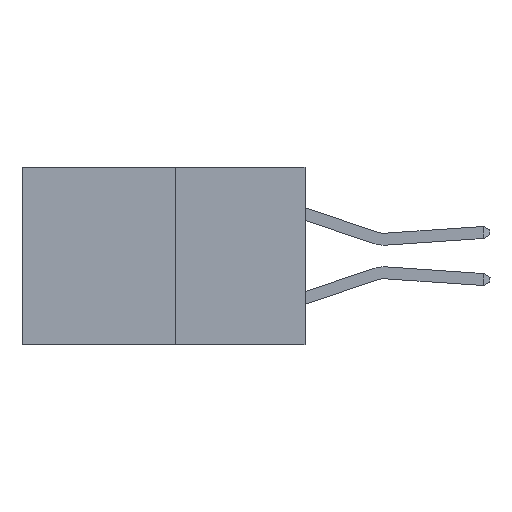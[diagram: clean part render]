
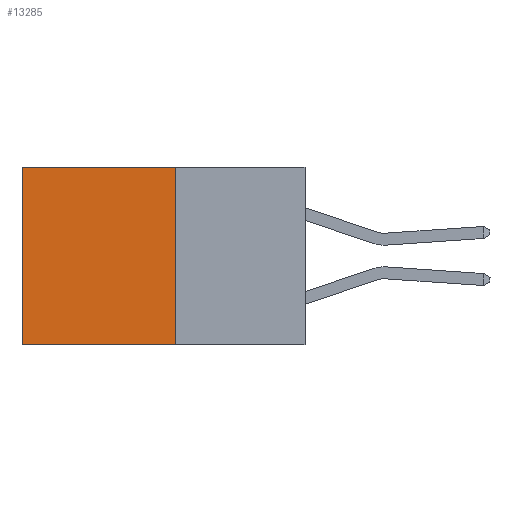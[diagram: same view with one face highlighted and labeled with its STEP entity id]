
A CAD part, left-side view. The second image highlights one B-rep face of the part: STEP entity #13285.
In plain terms, the highlighted planar face has unit normal (-1, 0, 0).
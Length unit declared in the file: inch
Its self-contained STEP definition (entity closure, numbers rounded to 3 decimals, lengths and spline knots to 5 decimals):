
#736 = ORIENTED_EDGE ( 'NONE', *, *, #5161, .F. ) ;
#1628 = PLANE ( 'NONE',  #15658 ) ;
#1926 = CARTESIAN_POINT ( 'NONE',  ( 0.277, 0.59, -0.37 ) ) ;
#3054 = FACE_OUTER_BOUND ( 'NONE', #21826, .T. ) ;
#3235 = VECTOR ( 'NONE', #4807, 39.37008 ) ;
#4187 = VERTEX_POINT ( 'NONE', #1926 ) ;
#4800 = CARTESIAN_POINT ( 'NONE',  ( 0.277, 0.27, -0.37 ) ) ;
#4807 = DIRECTION ( 'NONE',  ( 0., 0., -1. ) ) ;
#5161 = EDGE_CURVE ( 'NONE', #14429, #4187, #18227, .T. ) ;
#7952 = EDGE_CURVE ( 'NONE', #21503, #14429, #8270, .T. ) ;
#8237 = ORIENTED_EDGE ( 'NONE', *, *, #9964, .T. ) ;
#8270 = LINE ( 'NONE', #4800, #3235 ) ;
#8458 = DIRECTION ( 'NONE',  ( 0., 0., -1. ) ) ;
#8655 = VECTOR ( 'NONE', #10369, 39.37008 ) ;
#9775 = VECTOR ( 'NONE', #21558, 39.37008 ) ;
#9791 = CARTESIAN_POINT ( 'NONE',  ( 0.277, 0.27, 0. ) ) ;
#9964 = EDGE_CURVE ( 'NONE', #19637, #4187, #15143, .T. ) ;
#10276 = CARTESIAN_POINT ( 'NONE',  ( 0.277, 0.27, -0.37 ) ) ;
#10369 = DIRECTION ( 'NONE',  ( 0., 1., 0. ) ) ;
#12309 = ORIENTED_EDGE ( 'NONE', *, *, #16398, .T. ) ;
#13115 = ORIENTED_EDGE ( 'NONE', *, *, #7952, .F. ) ;
#13167 = CARTESIAN_POINT ( 'NONE',  ( 0.277, 0.59, 0. ) ) ;
#13285 = ADVANCED_FACE ( 'NONE', ( #3054 ), #1628, .F. ) ;
#13420 = CARTESIAN_POINT ( 'NONE',  ( 0.277, 0.59, -0.37 ) ) ;
#14429 = VERTEX_POINT ( 'NONE', #16674 ) ;
#14598 = VECTOR ( 'NONE', #18620, 39.37008 ) ;
#15143 = LINE ( 'NONE', #13420, #14598 ) ;
#15658 = AXIS2_PLACEMENT_3D ( 'NONE', #16954, #18629, #8458 ) ;
#16398 = EDGE_CURVE ( 'NONE', #21503, #19637, #17772, .T. ) ;
#16674 = CARTESIAN_POINT ( 'NONE',  ( 0.277, 0.27, -0.37 ) ) ;
#16954 = CARTESIAN_POINT ( 'NONE',  ( 0.277, 0.27, -0.37 ) ) ;
#17772 = LINE ( 'NONE', #9791, #9775 ) ;
#18227 = LINE ( 'NONE', #10276, #8655 ) ;
#18620 = DIRECTION ( 'NONE',  ( 0., 0., -1. ) ) ;
#18629 = DIRECTION ( 'NONE',  ( 1., 0., 0. ) ) ;
#19637 = VERTEX_POINT ( 'NONE', #13167 ) ;
#21503 = VERTEX_POINT ( 'NONE', #21612 ) ;
#21558 = DIRECTION ( 'NONE',  ( 0., 1., 0. ) ) ;
#21612 = CARTESIAN_POINT ( 'NONE',  ( 0.277, 0.27, 0. ) ) ;
#21826 = EDGE_LOOP ( 'NONE', ( #8237, #736, #13115, #12309 ) ) ;
